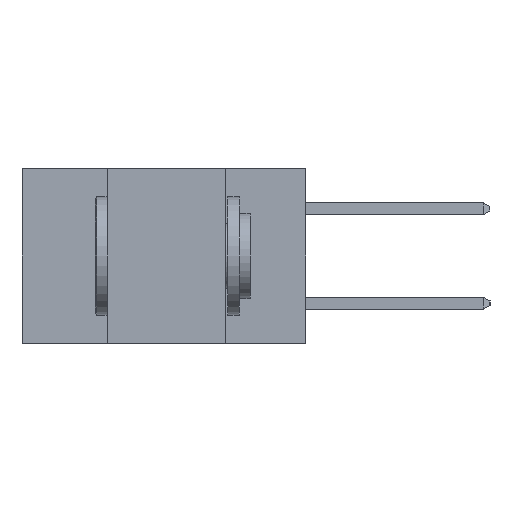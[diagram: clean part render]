
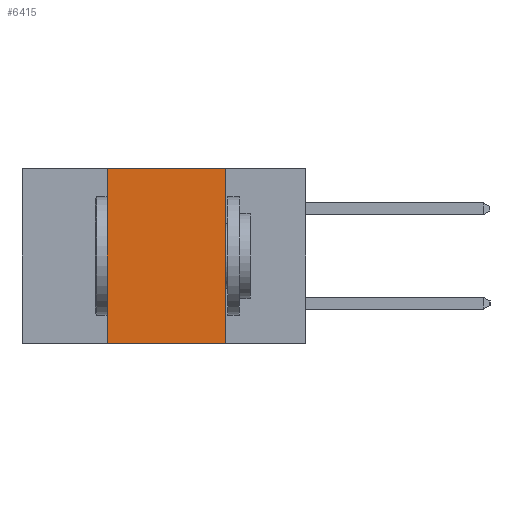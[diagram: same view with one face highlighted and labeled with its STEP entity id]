
A CAD part, left-side view. The second image highlights one B-rep face of the part: STEP entity #6415.
In plain terms, the highlighted planar face has unit normal (-1, 0, 0).
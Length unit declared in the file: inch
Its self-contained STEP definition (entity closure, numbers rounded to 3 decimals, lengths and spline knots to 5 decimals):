
#317 = DIRECTION ( 'NONE',  ( 0., 0., -1. ) ) ;
#873 = PLANE ( 'NONE',  #12371 ) ;
#1752 = LINE ( 'NONE', #12661, #13750 ) ;
#2117 = LINE ( 'NONE', #7512, #13768 ) ;
#2237 = CARTESIAN_POINT ( 'NONE',  ( 0., 0.17, -0.37 ) ) ;
#2372 = CARTESIAN_POINT ( 'NONE',  ( 0., 0.17, -0.37 ) ) ;
#2423 = DIRECTION ( 'NONE',  ( 0., 0., -1. ) ) ;
#2462 = VECTOR ( 'NONE', #5281, 39.37008 ) ;
#2833 = DIRECTION ( 'NONE',  ( 1., 0., 0. ) ) ;
#2972 = VERTEX_POINT ( 'NONE', #9669 ) ;
#3752 = CARTESIAN_POINT ( 'NONE',  ( 0., 0.17, 0. ) ) ;
#5281 = DIRECTION ( 'NONE',  ( 0., 0., 1. ) ) ;
#5510 = CARTESIAN_POINT ( 'NONE',  ( 0., 0.42, 0. ) ) ;
#5576 = VERTEX_POINT ( 'NONE', #2237 ) ;
#6071 = EDGE_CURVE ( 'NONE', #13656, #14008, #1752, .T. ) ;
#6113 = CARTESIAN_POINT ( 'NONE',  ( 0., 0.6, 0. ) ) ;
#6415 = ADVANCED_FACE ( 'NONE', ( #9243 ), #873, .F. ) ;
#7231 = DIRECTION ( 'NONE',  ( 0., -1., 0. ) ) ;
#7512 = CARTESIAN_POINT ( 'NONE',  ( 0., 0.6, -0.37 ) ) ;
#8957 = EDGE_LOOP ( 'NONE', ( #11908, #10546, #10366, #13277 ) ) ;
#9243 = FACE_OUTER_BOUND ( 'NONE', #8957, .T. ) ;
#9669 = CARTESIAN_POINT ( 'NONE',  ( 0., 0.42, -0.37 ) ) ;
#10366 = ORIENTED_EDGE ( 'NONE', *, *, #13720, .F. ) ;
#10546 = ORIENTED_EDGE ( 'NONE', *, *, #6071, .F. ) ;
#11908 = ORIENTED_EDGE ( 'NONE', *, *, #13502, .F. ) ;
#12371 = AXIS2_PLACEMENT_3D ( 'NONE', #6113, #2833, #317 ) ;
#12661 = CARTESIAN_POINT ( 'NONE',  ( 0., 0.6, 0. ) ) ;
#12685 = DIRECTION ( 'NONE',  ( 0., -1., 0. ) ) ;
#13277 = ORIENTED_EDGE ( 'NONE', *, *, #13291, .T. ) ;
#13291 = EDGE_CURVE ( 'NONE', #2972, #5576, #2117, .T. ) ;
#13502 = EDGE_CURVE ( 'NONE', #14008, #5576, #13940, .T. ) ;
#13595 = VECTOR ( 'NONE', #2423, 39.37008 ) ;
#13656 = VERTEX_POINT ( 'NONE', #5510 ) ;
#13720 = EDGE_CURVE ( 'NONE', #2972, #13656, #13754, .T. ) ;
#13750 = VECTOR ( 'NONE', #12685, 39.37008 ) ;
#13754 = LINE ( 'NONE', #13993, #2462 ) ;
#13768 = VECTOR ( 'NONE', #7231, 39.37008 ) ;
#13940 = LINE ( 'NONE', #2372, #13595 ) ;
#13993 = CARTESIAN_POINT ( 'NONE',  ( 0., 0.42, -0.37 ) ) ;
#14008 = VERTEX_POINT ( 'NONE', #3752 ) ;
